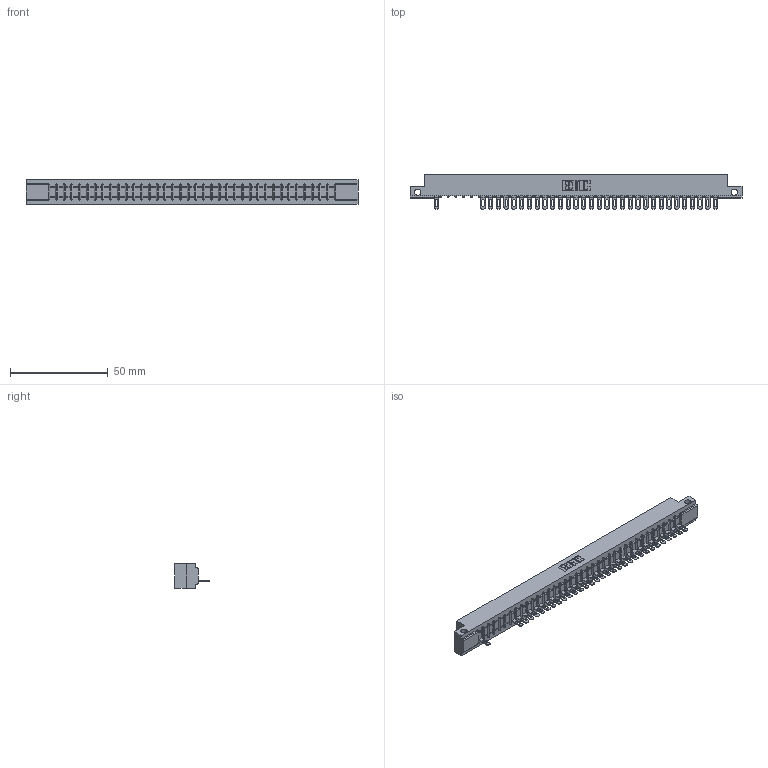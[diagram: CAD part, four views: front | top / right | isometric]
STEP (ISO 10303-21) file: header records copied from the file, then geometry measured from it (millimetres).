
FILE_DESCRIPTION (( 'STEP AP203' ), '1' );
FILE_NAME ('357-037-501-112.STEP', '2018-08-10T07:44:35', ( '' ), ( '' ), 'SwSTEP 2.0', 'SolidWorks 2016', '' );
FILE_SCHEMA (( 'CONFIG_CONTROL_DESIGN' ));
Length unit declared in the file: inch
Products named in the file (3): 307 Part_.128 Dia Side Mounting Holes; 307-290-002_501; 357-037-501-112
Assembly tree (33 placements, depth 2):
  357-037-501-112
    307 Part_.128 Dia Side Mounting Holes
    307-290-002_501  x32
Bounding box: 169.62 x 17.42 x 12.7 mm (x, y, z)
Volume: 17855.4 mm3; surface area: 21619.6 mm2
Topology: 33 solids, 33 shells, 2688 faces, 8259 edges, 5402 vertices
Faces by surface type: plane 1538, cylinder 1074, sphere 76
Entity records: 32972 total; most frequent: CARTESIAN_POINT 5583, ORIENTED_EDGE 5578, DIRECTION 5425, EDGE_CURVE 2789, VECTOR 2129, LINE 2129, VERTEX_POINT 1806, AXIS2_PLACEMENT_3D 1648
